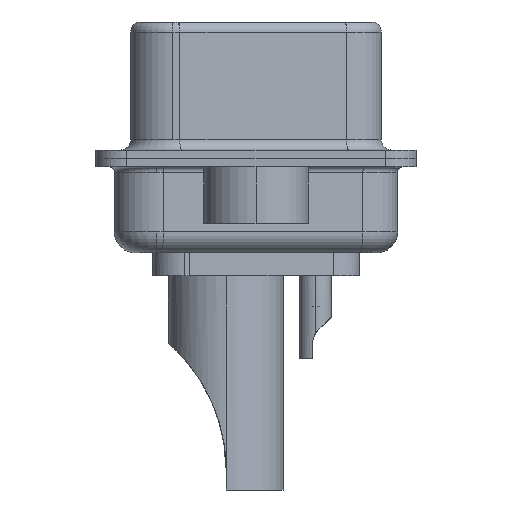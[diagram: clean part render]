
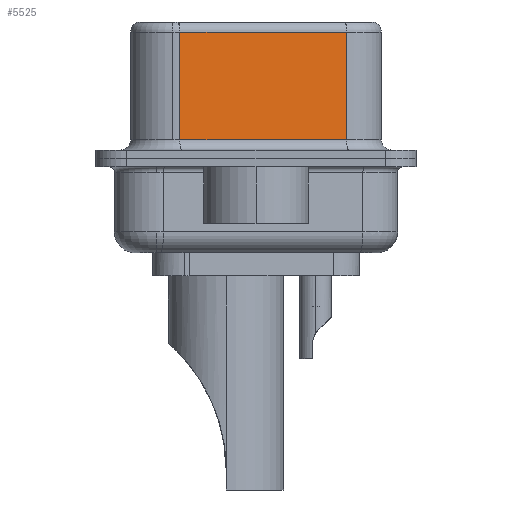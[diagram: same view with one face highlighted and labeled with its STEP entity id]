
A CAD part, left-side view. The second image highlights one B-rep face of the part: STEP entity #5525.
In plain terms, the highlighted planar face has unit normal (-0.985, -0.174, 0).
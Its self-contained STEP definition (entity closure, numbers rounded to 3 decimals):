
#204 = ORIENTED_EDGE ( 'NONE', *, *, #7374, .T. ) ;
#279 = VECTOR ( 'NONE', #24448, 1000. ) ;
#623 = LINE ( 'NONE', #2099, #16418 ) ;
#1952 = CARTESIAN_POINT ( 'NONE',  ( 3.73, 3.628, 0.9 ) ) ;
#2099 = CARTESIAN_POINT ( 'NONE',  ( 3.73, 3.628, 6.52 ) ) ;
#2499 = CARTESIAN_POINT ( 'NONE',  ( 5.132, -4.322, 6.02 ) ) ;
#3647 = VECTOR ( 'NONE', #6650, 1000. ) ;
#5525 = ADVANCED_FACE ( 'NONE', ( #22275 ), #7997, .F. ) ;
#6650 = DIRECTION ( 'NONE',  ( -0.174, 0.985, 0. ) ) ;
#7374 = EDGE_CURVE ( 'NONE', #17343, #20282, #623, .T. ) ;
#7472 = VERTEX_POINT ( 'NONE', #14670 ) ;
#7677 = EDGE_CURVE ( 'NONE', #7472, #25986, #11217, .T. ) ;
#7997 = PLANE ( 'NONE',  #13402 ) ;
#8154 = LINE ( 'NONE', #14251, #12308 ) ;
#9048 = LINE ( 'NONE', #2499, #3647 ) ;
#10045 = DIRECTION ( 'NONE',  ( -0.174, 0.985, 0. ) ) ;
#10175 = DIRECTION ( 'NONE',  ( 0.174, -0.985, 0. ) ) ;
#10223 = DIRECTION ( 'NONE',  ( 0., 0., -1. ) ) ;
#11217 = LINE ( 'NONE', #22396, #279 ) ;
#11954 = ORIENTED_EDGE ( 'NONE', *, *, #22363, .T. ) ;
#12308 = VECTOR ( 'NONE', #10175, 1000. ) ;
#13402 = AXIS2_PLACEMENT_3D ( 'NONE', #18252, #16201, #10045 ) ;
#14070 = CARTESIAN_POINT ( 'NONE',  ( 3.73, 3.628, 6.02 ) ) ;
#14251 = CARTESIAN_POINT ( 'NONE',  ( 5.132, -4.322, 0.9 ) ) ;
#14670 = CARTESIAN_POINT ( 'NONE',  ( 5.132, -4.322, 6.02 ) ) ;
#16201 = DIRECTION ( 'NONE',  ( 0.985, 0.174, 0. ) ) ;
#16418 = VECTOR ( 'NONE', #10223, 1000. ) ;
#16726 = CARTESIAN_POINT ( 'NONE',  ( 5.132, -4.322, 0.9 ) ) ;
#17343 = VERTEX_POINT ( 'NONE', #14070 ) ;
#18252 = CARTESIAN_POINT ( 'NONE',  ( 5.132, -4.322, 6.52 ) ) ;
#19545 = ORIENTED_EDGE ( 'NONE', *, *, #20286, .T. ) ;
#20282 = VERTEX_POINT ( 'NONE', #1952 ) ;
#20286 = EDGE_CURVE ( 'NONE', #20282, #25986, #8154, .T. ) ;
#20374 = ORIENTED_EDGE ( 'NONE', *, *, #7677, .F. ) ;
#22275 = FACE_OUTER_BOUND ( 'NONE', #25648, .T. ) ;
#22363 = EDGE_CURVE ( 'NONE', #7472, #17343, #9048, .T. ) ;
#22396 = CARTESIAN_POINT ( 'NONE',  ( 5.132, -4.322, 6.52 ) ) ;
#24448 = DIRECTION ( 'NONE',  ( 0., 0., -1. ) ) ;
#25648 = EDGE_LOOP ( 'NONE', ( #20374, #11954, #204, #19545 ) ) ;
#25986 = VERTEX_POINT ( 'NONE', #16726 ) ;
